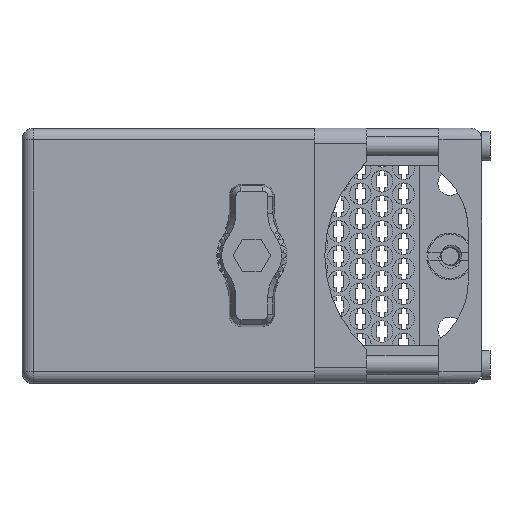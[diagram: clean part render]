
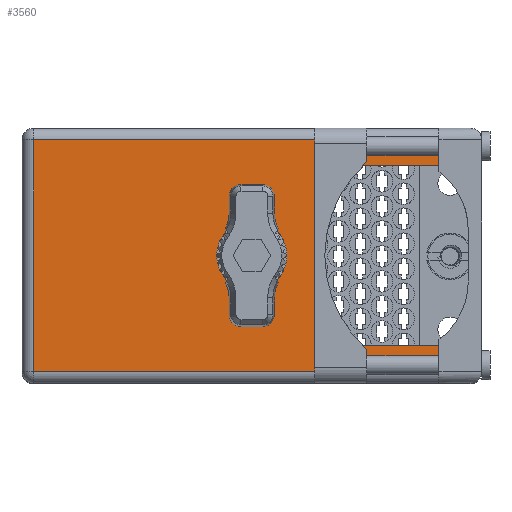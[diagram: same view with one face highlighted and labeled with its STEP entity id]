
A CAD part, top view. The second image highlights one B-rep face of the part: STEP entity #3560.
In plain terms, the highlighted face is planar.
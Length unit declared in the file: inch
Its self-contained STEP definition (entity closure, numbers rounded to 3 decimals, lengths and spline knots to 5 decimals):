
#1906 = LINE ( 'NONE', #11562, #76529 ) ;
#3295 = DIRECTION ( 'NONE',  ( 0., 1., 0. ) ) ;
#3359 = CARTESIAN_POINT ( 'NONE',  ( 2.499, 2.03, -1.305 ) ) ;
#3560 = ADVANCED_FACE ( 'NONE', ( #87521, #73898 ), #11700, .T. ) ;
#4523 = DIRECTION ( 'NONE',  ( 0., 0., 1. ) ) ;
#5349 = CARTESIAN_POINT ( 'NONE',  ( 1.785, 2.03, -0.225 ) ) ;
#7434 = DIRECTION ( 'NONE',  ( 0., 1., 0. ) ) ;
#7688 = DIRECTION ( 'NONE',  ( 0., 0., 1. ) ) ;
#7874 = VERTEX_POINT ( 'NONE', #5349 ) ;
#9852 = ORIENTED_EDGE ( 'NONE', *, *, #35745, .F. ) ;
#11415 = EDGE_CURVE ( 'NONE', #86172, #73908, #14411, .T. ) ;
#11562 = CARTESIAN_POINT ( 'NONE',  ( 2.499, 2.03, -0.225 ) ) ;
#11700 = PLANE ( 'NONE',  #105362 ) ;
#13444 = VECTOR ( 'NONE', #60946, 39.37008 ) ;
#13798 = DIRECTION ( 'NONE',  ( 0., 0., 1. ) ) ;
#14411 = CIRCLE ( 'NONE', #105841, 0.17 ) ;
#14616 = CARTESIAN_POINT ( 'NONE',  ( 1.3775, 2.03, -0.765 ) ) ;
#15830 = EDGE_CURVE ( 'NONE', #32636, #16354, #50542, .T. ) ;
#16354 = VERTEX_POINT ( 'NONE', #19182 ) ;
#19182 = CARTESIAN_POINT ( 'NONE',  ( 0.07, 2.03, -1.46 ) ) ;
#19657 = CARTESIAN_POINT ( 'NONE',  ( 1.3775, 2.03, -0.935 ) ) ;
#20030 = CARTESIAN_POINT ( 'NONE',  ( 0., 2.03, -1.53 ) ) ;
#20249 = VECTOR ( 'NONE', #4523, 39.37008 ) ;
#20271 = DIRECTION ( 'NONE',  ( -1., 0., 0. ) ) ;
#21820 = CARTESIAN_POINT ( 'NONE',  ( 1.3775, 2.03, -0.595 ) ) ;
#22133 = EDGE_CURVE ( 'NONE', #88277, #80428, #70133, .T. ) ;
#22993 = LINE ( 'NONE', #56954, #112496 ) ;
#23323 = VECTOR ( 'NONE', #7688, 39.37008 ) ;
#23360 = ORIENTED_EDGE ( 'NONE', *, *, #86259, .F. ) ;
#24117 = EDGE_LOOP ( 'NONE', ( #81974, #23360 ) ) ;
#25511 = EDGE_CURVE ( 'NONE', #16354, #88277, #46337, .T. ) ;
#25804 = LINE ( 'NONE', #48237, #107151 ) ;
#25993 = VERTEX_POINT ( 'NONE', #67435 ) ;
#28156 = VECTOR ( 'NONE', #30042, 39.37008 ) ;
#30042 = DIRECTION ( 'NONE',  ( 1., 0., 0. ) ) ;
#32636 = VERTEX_POINT ( 'NONE', #99267 ) ;
#34872 = CARTESIAN_POINT ( 'NONE',  ( 0., 2.03, -1.46 ) ) ;
#34950 = CARTESIAN_POINT ( 'NONE',  ( 2.499, 2.03, -0.225 ) ) ;
#35164 = CARTESIAN_POINT ( 'NONE',  ( 1.785, 2.03, -1.305 ) ) ;
#35376 = CARTESIAN_POINT ( 'NONE',  ( 0.07, 2.03, -0.07 ) ) ;
#35745 = EDGE_CURVE ( 'NONE', #73250, #80428, #51485, .T. ) ;
#36606 = ORIENTED_EDGE ( 'NONE', *, *, #15830, .T. ) ;
#39672 = ORIENTED_EDGE ( 'NONE', *, *, #25511, .T. ) ;
#46337 = LINE ( 'NONE', #69395, #23323 ) ;
#46713 = CARTESIAN_POINT ( 'NONE',  ( 2.499, 2.03, -0.07 ) ) ;
#48237 = CARTESIAN_POINT ( 'NONE',  ( 2.499, 2.03, -1.53 ) ) ;
#48625 = LINE ( 'NONE', #35164, #13444 ) ;
#50542 = LINE ( 'NONE', #34872, #55956 ) ;
#51485 = LINE ( 'NONE', #82976, #20249 ) ;
#55956 = VECTOR ( 'NONE', #61022, 39.37008 ) ;
#56954 = CARTESIAN_POINT ( 'NONE',  ( 2.499, 2.03, -1.305 ) ) ;
#59214 = EDGE_CURVE ( 'NONE', #32636, #104495, #25804, .T. ) ;
#60946 = DIRECTION ( 'NONE',  ( 0., 0., -1. ) ) ;
#61022 = DIRECTION ( 'NONE',  ( -1., 0., 0. ) ) ;
#64292 = DIRECTION ( 'NONE',  ( 0., 0., 1. ) ) ;
#67435 = CARTESIAN_POINT ( 'NONE',  ( 1.785, 2.03, -1.305 ) ) ;
#69395 = CARTESIAN_POINT ( 'NONE',  ( 0.07, 2.03, -1.53 ) ) ;
#70133 = LINE ( 'NONE', #46713, #28156 ) ;
#73250 = VERTEX_POINT ( 'NONE', #34950 ) ;
#73898 = FACE_BOUND ( 'NONE', #24117, .T. ) ;
#73908 = VERTEX_POINT ( 'NONE', #19657 ) ;
#75018 = ORIENTED_EDGE ( 'NONE', *, *, #22133, .T. ) ;
#75121 = DIRECTION ( 'NONE',  ( 1., 0., 0. ) ) ;
#76529 = VECTOR ( 'NONE', #20271, 39.37008 ) ;
#77335 = ORIENTED_EDGE ( 'NONE', *, *, #79194, .T. ) ;
#79194 = EDGE_CURVE ( 'NONE', #25993, #104495, #22993, .T. ) ;
#80428 = VERTEX_POINT ( 'NONE', #97938 ) ;
#80709 = DIRECTION ( 'NONE',  ( 0., 1., 0. ) ) ;
#81601 = CIRCLE ( 'NONE', #105061, 0.17 ) ;
#81974 = ORIENTED_EDGE ( 'NONE', *, *, #11415, .F. ) ;
#82342 = EDGE_CURVE ( 'NONE', #73250, #7874, #1906, .T. ) ;
#82976 = CARTESIAN_POINT ( 'NONE',  ( 2.499, 2.03, -1.53 ) ) ;
#83840 = ORIENTED_EDGE ( 'NONE', *, *, #88849, .T. ) ;
#86172 = VERTEX_POINT ( 'NONE', #21820 ) ;
#86259 = EDGE_CURVE ( 'NONE', #73908, #86172, #81601, .T. ) ;
#87521 = FACE_OUTER_BOUND ( 'NONE', #93541, .T. ) ;
#88277 = VERTEX_POINT ( 'NONE', #35376 ) ;
#88849 = EDGE_CURVE ( 'NONE', #7874, #25993, #48625, .T. ) ;
#90080 = CARTESIAN_POINT ( 'NONE',  ( 1.3775, 2.03, -0.765 ) ) ;
#93541 = EDGE_LOOP ( 'NONE', ( #39672, #75018, #9852, #103869, #83840, #77335, #107113, #36606 ) ) ;
#97938 = CARTESIAN_POINT ( 'NONE',  ( 2.499, 2.03, -0.07 ) ) ;
#98082 = DIRECTION ( 'NONE',  ( 0., 0., 1. ) ) ;
#99267 = CARTESIAN_POINT ( 'NONE',  ( 2.499, 2.03, -1.46 ) ) ;
#101395 = DIRECTION ( 'NONE',  ( 0., 0., 1. ) ) ;
#103869 = ORIENTED_EDGE ( 'NONE', *, *, #82342, .T. ) ;
#104495 = VERTEX_POINT ( 'NONE', #3359 ) ;
#105061 = AXIS2_PLACEMENT_3D ( 'NONE', #14616, #7434, #101395 ) ;
#105362 = AXIS2_PLACEMENT_3D ( 'NONE', #20030, #80709, #98082 ) ;
#105841 = AXIS2_PLACEMENT_3D ( 'NONE', #90080, #3295, #64292 ) ;
#107113 = ORIENTED_EDGE ( 'NONE', *, *, #59214, .F. ) ;
#107151 = VECTOR ( 'NONE', #13798, 39.37008 ) ;
#112496 = VECTOR ( 'NONE', #75121, 39.37008 ) ;
